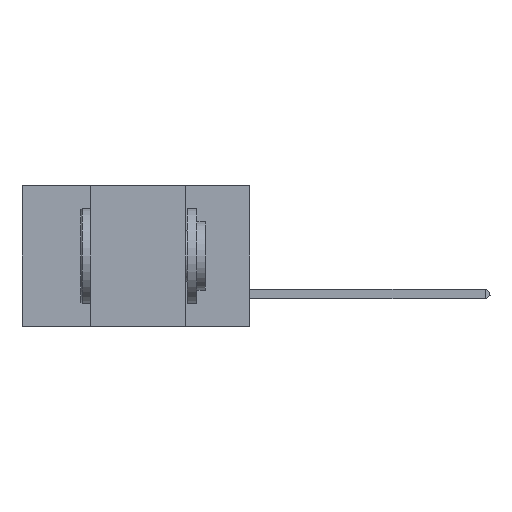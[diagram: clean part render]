
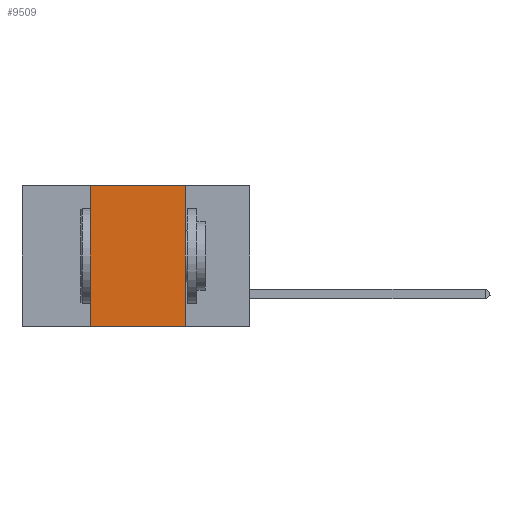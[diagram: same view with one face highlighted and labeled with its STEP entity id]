
A CAD part, left-side view. The second image highlights one B-rep face of the part: STEP entity #9509.
In plain terms, the highlighted planar face has unit normal (-1, 0, 0).
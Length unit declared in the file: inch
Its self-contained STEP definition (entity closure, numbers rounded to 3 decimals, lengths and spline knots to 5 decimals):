
#2201 = EDGE_CURVE ( 'NONE', #32231, #5460, #26212, .T. ) ;
#2373 = LINE ( 'NONE', #10593, #14481 ) ;
#4203 = DIRECTION ( 'NONE',  ( 0., 0., -1. ) ) ;
#5460 = VERTEX_POINT ( 'NONE', #24908 ) ;
#5698 = ORIENTED_EDGE ( 'NONE', *, *, #2201, .F. ) ;
#6476 = ORIENTED_EDGE ( 'NONE', *, *, #32123, .F. ) ;
#7158 = EDGE_CURVE ( 'NONE', #5460, #30426, #20218, .T. ) ;
#7858 = VECTOR ( 'NONE', #14187, 39.37008 ) ;
#8325 = LINE ( 'NONE', #11954, #21600 ) ;
#9509 = ADVANCED_FACE ( 'NONE', ( #11883 ), #31615, .F. ) ;
#10593 = CARTESIAN_POINT ( 'NONE',  ( 0., 0.17, 0. ) ) ;
#11137 = CARTESIAN_POINT ( 'NONE',  ( 0., 0.6, 0. ) ) ;
#11786 = VERTEX_POINT ( 'NONE', #19858 ) ;
#11883 = FACE_OUTER_BOUND ( 'NONE', #31993, .T. ) ;
#11954 = CARTESIAN_POINT ( 'NONE',  ( 0., 0.6, -0.37 ) ) ;
#13206 = ORIENTED_EDGE ( 'NONE', *, *, #7158, .F. ) ;
#14187 = DIRECTION ( 'NONE',  ( 0., 0., 1. ) ) ;
#14481 = VECTOR ( 'NONE', #25741, 39.37008 ) ;
#15470 = CARTESIAN_POINT ( 'NONE',  ( 0., 0.42, -0.37 ) ) ;
#15561 = CARTESIAN_POINT ( 'NONE',  ( 0., 0.17, 0. ) ) ;
#16138 = DIRECTION ( 'NONE',  ( 0., -1., 0. ) ) ;
#19858 = CARTESIAN_POINT ( 'NONE',  ( 0., 0.17, -0.37 ) ) ;
#20218 = LINE ( 'NONE', #11137, #30404 ) ;
#21308 = DIRECTION ( 'NONE',  ( 1., 0., 0. ) ) ;
#21600 = VECTOR ( 'NONE', #26997, 39.37008 ) ;
#22132 = EDGE_CURVE ( 'NONE', #32231, #11786, #8325, .T. ) ;
#24908 = CARTESIAN_POINT ( 'NONE',  ( 0., 0.42, 0. ) ) ;
#25741 = DIRECTION ( 'NONE',  ( 0., 0., -1. ) ) ;
#26004 = AXIS2_PLACEMENT_3D ( 'NONE', #26438, #21308, #4203 ) ;
#26212 = LINE ( 'NONE', #29150, #7858 ) ;
#26438 = CARTESIAN_POINT ( 'NONE',  ( 0., 0.6, 0. ) ) ;
#26997 = DIRECTION ( 'NONE',  ( 0., -1., 0. ) ) ;
#29150 = CARTESIAN_POINT ( 'NONE',  ( 0., 0.42, 0. ) ) ;
#30404 = VECTOR ( 'NONE', #16138, 39.37008 ) ;
#30426 = VERTEX_POINT ( 'NONE', #15561 ) ;
#31497 = ORIENTED_EDGE ( 'NONE', *, *, #22132, .T. ) ;
#31615 = PLANE ( 'NONE',  #26004 ) ;
#31993 = EDGE_LOOP ( 'NONE', ( #6476, #13206, #5698, #31497 ) ) ;
#32123 = EDGE_CURVE ( 'NONE', #30426, #11786, #2373, .T. ) ;
#32231 = VERTEX_POINT ( 'NONE', #15470 ) ;
